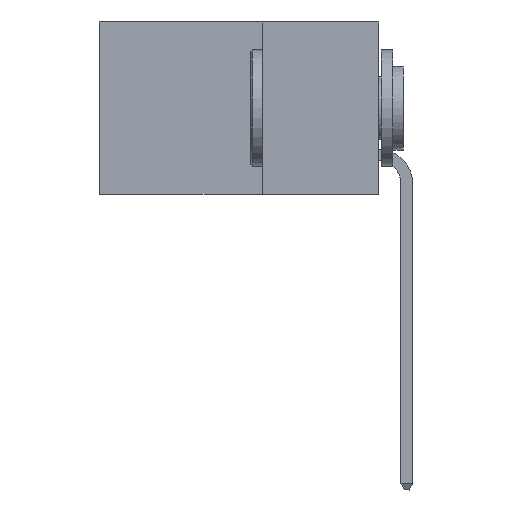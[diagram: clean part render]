
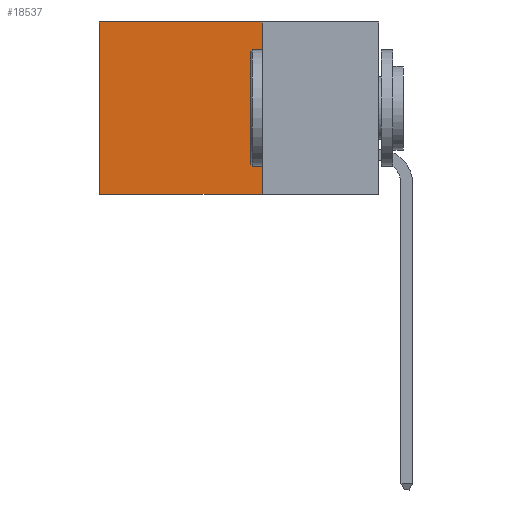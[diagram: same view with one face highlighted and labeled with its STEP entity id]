
A CAD part, left-side view. The second image highlights one B-rep face of the part: STEP entity #18537.
In plain terms, the highlighted planar face has unit normal (-1, 0, 0).
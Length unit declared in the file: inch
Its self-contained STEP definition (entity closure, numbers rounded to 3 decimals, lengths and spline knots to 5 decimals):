
#373 = CARTESIAN_POINT ( 'NONE',  ( 0.2615, 0.6, -0.37 ) ) ;
#534 = LINE ( 'NONE', #14080, #8021 ) ;
#1452 = CARTESIAN_POINT ( 'NONE',  ( 0.2615, 0.6, -0.37 ) ) ;
#1942 = VERTEX_POINT ( 'NONE', #3973 ) ;
#2496 = CARTESIAN_POINT ( 'NONE',  ( 0.2615, 0.25, -0.37 ) ) ;
#2740 = VERTEX_POINT ( 'NONE', #9100 ) ;
#3541 = EDGE_CURVE ( 'NONE', #2740, #11943, #12525, .T. ) ;
#3963 = ORIENTED_EDGE ( 'NONE', *, *, #18455, .F. ) ;
#3973 = CARTESIAN_POINT ( 'NONE',  ( 0.2615, 0.25, -0.37 ) ) ;
#5041 = CARTESIAN_POINT ( 'NONE',  ( 0.2615, 0.25, 0. ) ) ;
#5457 = CARTESIAN_POINT ( 'NONE',  ( 0.2615, 0.25, 0. ) ) ;
#5594 = PLANE ( 'NONE',  #14698 ) ;
#7759 = LINE ( 'NONE', #10661, #15430 ) ;
#8021 = VECTOR ( 'NONE', #17072, 39.37008 ) ;
#8662 = ORIENTED_EDGE ( 'NONE', *, *, #3541, .T. ) ;
#8670 = EDGE_CURVE ( 'NONE', #1942, #11943, #7759, .T. ) ;
#9100 = CARTESIAN_POINT ( 'NONE',  ( 0.2615, 0.6, 0. ) ) ;
#9582 = ORIENTED_EDGE ( 'NONE', *, *, #8670, .F. ) ;
#10661 = CARTESIAN_POINT ( 'NONE',  ( 0.2615, 0.25, -0.37 ) ) ;
#10934 = DIRECTION ( 'NONE',  ( 0., 0., -1. ) ) ;
#11435 = VECTOR ( 'NONE', #10934, 39.37008 ) ;
#11442 = LINE ( 'NONE', #5457, #14557 ) ;
#11484 = FACE_OUTER_BOUND ( 'NONE', #12212, .T. ) ;
#11833 = EDGE_CURVE ( 'NONE', #16653, #2740, #11442, .T. ) ;
#11943 = VERTEX_POINT ( 'NONE', #1452 ) ;
#12212 = EDGE_LOOP ( 'NONE', ( #8662, #9582, #3963, #18600 ) ) ;
#12525 = LINE ( 'NONE', #373, #11435 ) ;
#12737 = DIRECTION ( 'NONE',  ( 0., 1., 0. ) ) ;
#14080 = CARTESIAN_POINT ( 'NONE',  ( 0.2615, 0.25, -0.37 ) ) ;
#14557 = VECTOR ( 'NONE', #12737, 39.37008 ) ;
#14698 = AXIS2_PLACEMENT_3D ( 'NONE', #2496, #19046, #18946 ) ;
#15430 = VECTOR ( 'NONE', #17140, 39.37008 ) ;
#16653 = VERTEX_POINT ( 'NONE', #5041 ) ;
#17072 = DIRECTION ( 'NONE',  ( 0., 0., -1. ) ) ;
#17140 = DIRECTION ( 'NONE',  ( 0., 1., 0. ) ) ;
#18455 = EDGE_CURVE ( 'NONE', #16653, #1942, #534, .T. ) ;
#18537 = ADVANCED_FACE ( 'NONE', ( #11484 ), #5594, .F. ) ;
#18600 = ORIENTED_EDGE ( 'NONE', *, *, #11833, .T. ) ;
#18946 = DIRECTION ( 'NONE',  ( 0., 0., -1. ) ) ;
#19046 = DIRECTION ( 'NONE',  ( 1., 0., 0. ) ) ;
